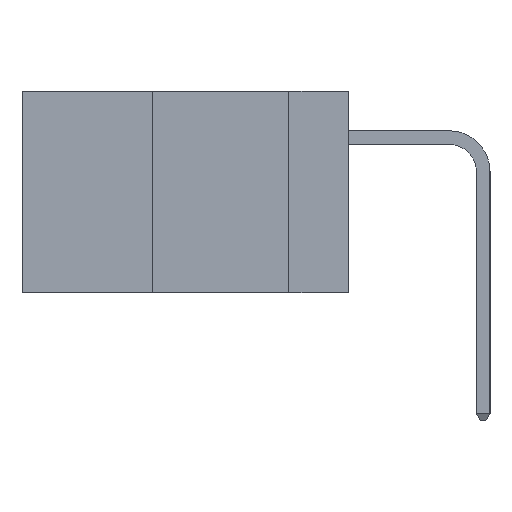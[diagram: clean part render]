
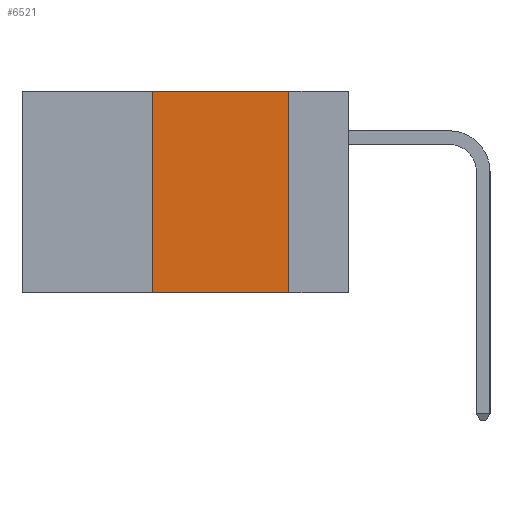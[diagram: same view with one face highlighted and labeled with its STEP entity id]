
A CAD part, left-side view. The second image highlights one B-rep face of the part: STEP entity #6521.
In plain terms, the highlighted planar face has unit normal (-1, 0, 0).
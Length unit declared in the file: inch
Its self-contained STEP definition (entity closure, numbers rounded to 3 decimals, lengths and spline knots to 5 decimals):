
#141 = VERTEX_POINT ( 'NONE', #2220 ) ;
#447 = EDGE_CURVE ( 'NONE', #1414, #2631, #450, .T. ) ;
#450 = LINE ( 'NONE', #6094, #11288 ) ;
#730 = ORIENTED_EDGE ( 'NONE', *, *, #5464, .F. ) ;
#937 = DIRECTION ( 'NONE',  ( 0., -1., 0. ) ) ;
#1081 = VECTOR ( 'NONE', #937, 39.37008 ) ;
#1414 = VERTEX_POINT ( 'NONE', #6607 ) ;
#1516 = CARTESIAN_POINT ( 'NONE',  ( 0., 0.6, -0.37 ) ) ;
#1988 = CARTESIAN_POINT ( 'NONE',  ( 0., 0.11, 0. ) ) ;
#2220 = CARTESIAN_POINT ( 'NONE',  ( 0., 0.11, -0.37 ) ) ;
#2414 = DIRECTION ( 'NONE',  ( 0., -1., 0. ) ) ;
#2631 = VERTEX_POINT ( 'NONE', #9511 ) ;
#2802 = DIRECTION ( 'NONE',  ( 0., 0., -1. ) ) ;
#3670 = VERTEX_POINT ( 'NONE', #7459 ) ;
#4052 = EDGE_CURVE ( 'NONE', #2631, #3670, #10411, .T. ) ;
#4526 = EDGE_LOOP ( 'NONE', ( #730, #5472, #7751, #10088 ) ) ;
#4663 = LINE ( 'NONE', #1988, #7238 ) ;
#4699 = AXIS2_PLACEMENT_3D ( 'NONE', #7161, #8024, #2802 ) ;
#5132 = EDGE_CURVE ( 'NONE', #1414, #141, #11038, .T. ) ;
#5464 = EDGE_CURVE ( 'NONE', #3670, #141, #4663, .T. ) ;
#5472 = ORIENTED_EDGE ( 'NONE', *, *, #4052, .F. ) ;
#5664 = DIRECTION ( 'NONE',  ( 0., 0., 1. ) ) ;
#6094 = CARTESIAN_POINT ( 'NONE',  ( 0., 0.36, 0. ) ) ;
#6291 = PLANE ( 'NONE',  #4699 ) ;
#6396 = DIRECTION ( 'NONE',  ( 0., 0., -1. ) ) ;
#6446 = VECTOR ( 'NONE', #2414, 39.37008 ) ;
#6521 = ADVANCED_FACE ( 'NONE', ( #11257 ), #6291, .F. ) ;
#6607 = CARTESIAN_POINT ( 'NONE',  ( 0., 0.36, -0.37 ) ) ;
#7161 = CARTESIAN_POINT ( 'NONE',  ( 0., 0.6, 0. ) ) ;
#7238 = VECTOR ( 'NONE', #6396, 39.37008 ) ;
#7459 = CARTESIAN_POINT ( 'NONE',  ( 0., 0.11, 0. ) ) ;
#7751 = ORIENTED_EDGE ( 'NONE', *, *, #447, .F. ) ;
#8024 = DIRECTION ( 'NONE',  ( 1., 0., 0. ) ) ;
#9511 = CARTESIAN_POINT ( 'NONE',  ( 0., 0.36, 0. ) ) ;
#9694 = CARTESIAN_POINT ( 'NONE',  ( 0., 0.6, 0. ) ) ;
#10088 = ORIENTED_EDGE ( 'NONE', *, *, #5132, .T. ) ;
#10411 = LINE ( 'NONE', #9694, #1081 ) ;
#11038 = LINE ( 'NONE', #1516, #6446 ) ;
#11257 = FACE_OUTER_BOUND ( 'NONE', #4526, .T. ) ;
#11288 = VECTOR ( 'NONE', #5664, 39.37008 ) ;
